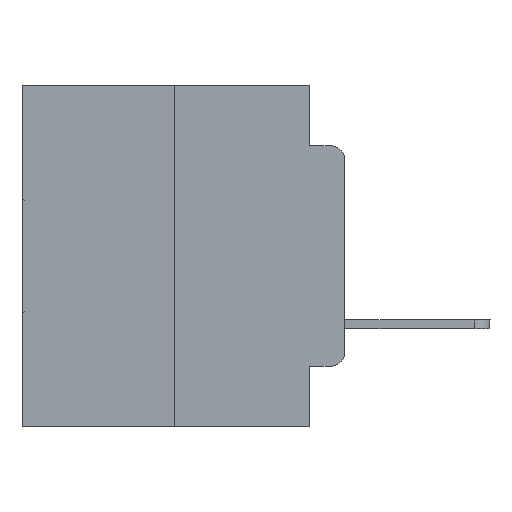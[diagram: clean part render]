
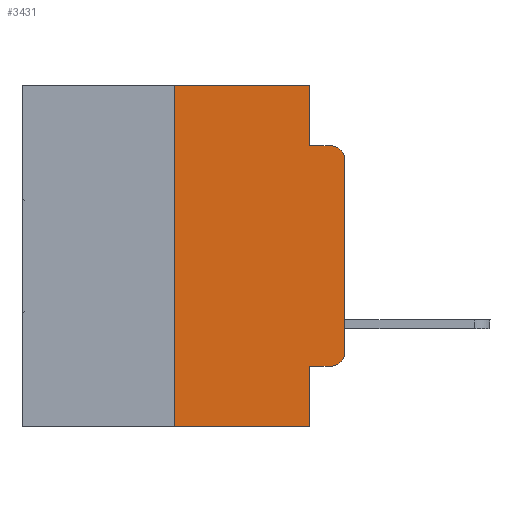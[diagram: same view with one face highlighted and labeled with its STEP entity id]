
A CAD part, left-side view. The second image highlights one B-rep face of the part: STEP entity #3431.
In plain terms, the highlighted planar face has unit normal (-1, 0, 0).
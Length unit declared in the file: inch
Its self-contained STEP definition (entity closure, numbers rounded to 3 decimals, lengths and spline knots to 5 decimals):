
#162 = DIRECTION ( 'NONE',  ( -1., 0., 0. ) ) ;
#295 = VERTEX_POINT ( 'NONE', #6868 ) ;
#637 = CARTESIAN_POINT ( 'NONE',  ( 0., 0.02, -0.4115 ) ) ;
#737 = VERTEX_POINT ( 'NONE', #6688 ) ;
#825 = EDGE_CURVE ( 'NONE', #737, #11321, #18460, .T. ) ;
#1387 = EDGE_CURVE ( 'NONE', #29007, #3425, #28203, .T. ) ;
#1582 = ORIENTED_EDGE ( 'NONE', *, *, #28420, .T. ) ;
#1652 = CARTESIAN_POINT ( 'NONE',  ( 0., 0., 0. ) ) ;
#2148 = VERTEX_POINT ( 'NONE', #12827 ) ;
#2608 = AXIS2_PLACEMENT_3D ( 'NONE', #13949, #18780, #27968 ) ;
#2728 = DIRECTION ( 'NONE',  ( 0., 0., 1. ) ) ;
#3110 = EDGE_CURVE ( 'NONE', #295, #2148, #27893, .T. ) ;
#3425 = VERTEX_POINT ( 'NONE', #10807 ) ;
#3431 = ADVANCED_FACE ( 'NONE', ( #24999 ), #16091, .F. ) ;
#3813 = LINE ( 'NONE', #12995, #10114 ) ;
#4442 = EDGE_CURVE ( 'NONE', #11321, #24416, #20964, .T. ) ;
#5596 = EDGE_CURVE ( 'NONE', #295, #3425, #11342, .T. ) ;
#5876 = CARTESIAN_POINT ( 'NONE',  ( 0., 0., -0.1085 ) ) ;
#6538 = DIRECTION ( 'NONE',  ( 0., 0., -1. ) ) ;
#6688 = CARTESIAN_POINT ( 'NONE',  ( 0., 0.051, 0. ) ) ;
#6868 = CARTESIAN_POINT ( 'NONE',  ( 0., 0.25, -0.5 ) ) ;
#7010 = EDGE_CURVE ( 'NONE', #14536, #13848, #26977, .T. ) ;
#7149 = LINE ( 'NONE', #20582, #23803 ) ;
#8207 = CARTESIAN_POINT ( 'NONE',  ( 0., 0., -0.3915 ) ) ;
#8684 = EDGE_LOOP ( 'NONE', ( #15167, #1582, #21241, #23757, #24203, #15164, #28158, #16300, #9314, #19852 ) ) ;
#9314 = ORIENTED_EDGE ( 'NONE', *, *, #9545, .T. ) ;
#9403 = DIRECTION ( 'NONE',  ( 0., -1., 0. ) ) ;
#9545 = EDGE_CURVE ( 'NONE', #29007, #17593, #3813, .T. ) ;
#9615 = VECTOR ( 'NONE', #29345, 39.37008 ) ;
#9991 = VECTOR ( 'NONE', #18153, 39.37008 ) ;
#10114 = VECTOR ( 'NONE', #17678, 39.37008 ) ;
#10807 = CARTESIAN_POINT ( 'NONE',  ( 0., 0.051, -0.5 ) ) ;
#11276 = VECTOR ( 'NONE', #16424, 39.37008 ) ;
#11321 = VERTEX_POINT ( 'NONE', #24684 ) ;
#11342 = LINE ( 'NONE', #27493, #9991 ) ;
#11814 = VECTOR ( 'NONE', #6538, 39.37008 ) ;
#12827 = CARTESIAN_POINT ( 'NONE',  ( 0., 0.25, 0. ) ) ;
#12995 = CARTESIAN_POINT ( 'NONE',  ( 0., 0.051, -0.4115 ) ) ;
#13191 = CARTESIAN_POINT ( 'NONE',  ( 0., 0.051, -0.4115 ) ) ;
#13232 = CARTESIAN_POINT ( 'NONE',  ( 0., 0.473, 0. ) ) ;
#13848 = VERTEX_POINT ( 'NONE', #5876 ) ;
#13949 = CARTESIAN_POINT ( 'NONE',  ( 0., 0.02, -0.3915 ) ) ;
#14168 = CARTESIAN_POINT ( 'NONE',  ( 0., 0.25, 0. ) ) ;
#14473 = CARTESIAN_POINT ( 'NONE',  ( 0., 0.051, 0. ) ) ;
#14536 = VERTEX_POINT ( 'NONE', #8207 ) ;
#15164 = ORIENTED_EDGE ( 'NONE', *, *, #3110, .F. ) ;
#15167 = ORIENTED_EDGE ( 'NONE', *, *, #7010, .T. ) ;
#15485 = DIRECTION ( 'NONE',  ( 1., 0., 0. ) ) ;
#16091 = PLANE ( 'NONE',  #19921 ) ;
#16300 = ORIENTED_EDGE ( 'NONE', *, *, #1387, .F. ) ;
#16424 = DIRECTION ( 'NONE',  ( 0., -1., 0. ) ) ;
#17593 = VERTEX_POINT ( 'NONE', #637 ) ;
#17678 = DIRECTION ( 'NONE',  ( 0., -1., 0. ) ) ;
#18153 = DIRECTION ( 'NONE',  ( 0., -1., 0. ) ) ;
#18460 = LINE ( 'NONE', #29754, #11814 ) ;
#18555 = DIRECTION ( 'NONE',  ( 0., 0., -1. ) ) ;
#18780 = DIRECTION ( 'NONE',  ( -1., 0., 0. ) ) ;
#19007 = CARTESIAN_POINT ( 'NONE',  ( 0., 0.051, -0.0885 ) ) ;
#19852 = ORIENTED_EDGE ( 'NONE', *, *, #29223, .T. ) ;
#19921 = AXIS2_PLACEMENT_3D ( 'NONE', #13232, #15485, #25144 ) ;
#20026 = CIRCLE ( 'NONE', #29662, 0.02 ) ;
#20582 = CARTESIAN_POINT ( 'NONE',  ( 0., 0.473, 0. ) ) ;
#20964 = LINE ( 'NONE', #19007, #11276 ) ;
#21241 = ORIENTED_EDGE ( 'NONE', *, *, #4442, .F. ) ;
#22755 = DIRECTION ( 'NONE',  ( 0., 0., 1. ) ) ;
#23757 = ORIENTED_EDGE ( 'NONE', *, *, #825, .F. ) ;
#23803 = VECTOR ( 'NONE', #9403, 39.37008 ) ;
#24203 = ORIENTED_EDGE ( 'NONE', *, *, #27941, .F. ) ;
#24416 = VERTEX_POINT ( 'NONE', #26090 ) ;
#24533 = VECTOR ( 'NONE', #22755, 39.37008 ) ;
#24684 = CARTESIAN_POINT ( 'NONE',  ( 0., 0.051, -0.0885 ) ) ;
#24999 = FACE_OUTER_BOUND ( 'NONE', #8684, .T. ) ;
#25144 = DIRECTION ( 'NONE',  ( 0., 0., -1. ) ) ;
#26061 = VECTOR ( 'NONE', #2728, 39.37008 ) ;
#26090 = CARTESIAN_POINT ( 'NONE',  ( 0., 0.02, -0.0885 ) ) ;
#26977 = LINE ( 'NONE', #1652, #24533 ) ;
#27493 = CARTESIAN_POINT ( 'NONE',  ( 0., 0.473, -0.5 ) ) ;
#27893 = LINE ( 'NONE', #14168, #26061 ) ;
#27941 = EDGE_CURVE ( 'NONE', #2148, #737, #7149, .T. ) ;
#27968 = DIRECTION ( 'NONE',  ( 0., 0., -1. ) ) ;
#28028 = CARTESIAN_POINT ( 'NONE',  ( 0., 0.02, -0.1085 ) ) ;
#28158 = ORIENTED_EDGE ( 'NONE', *, *, #5596, .T. ) ;
#28203 = LINE ( 'NONE', #14473, #9615 ) ;
#28420 = EDGE_CURVE ( 'NONE', #13848, #24416, #20026, .T. ) ;
#28595 = CIRCLE ( 'NONE', #2608, 0.02 ) ;
#29007 = VERTEX_POINT ( 'NONE', #13191 ) ;
#29223 = EDGE_CURVE ( 'NONE', #17593, #14536, #28595, .T. ) ;
#29345 = DIRECTION ( 'NONE',  ( 0., 0., -1. ) ) ;
#29662 = AXIS2_PLACEMENT_3D ( 'NONE', #28028, #162, #18555 ) ;
#29754 = CARTESIAN_POINT ( 'NONE',  ( 0., 0.051, 0. ) ) ;
